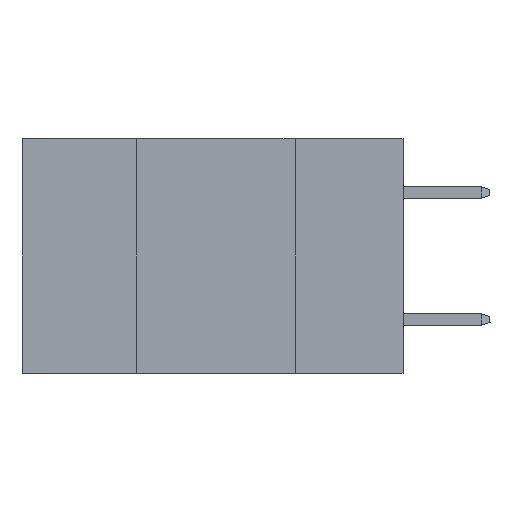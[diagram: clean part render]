
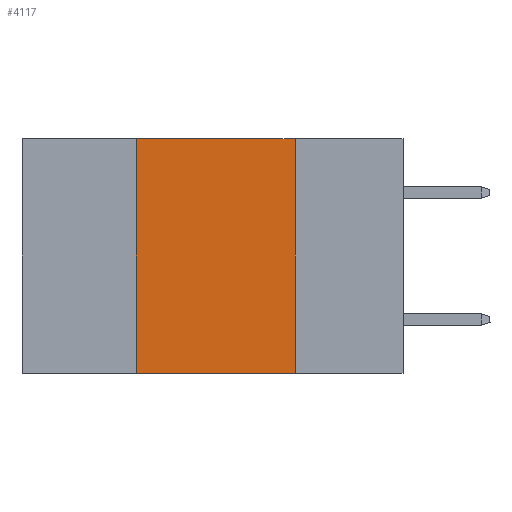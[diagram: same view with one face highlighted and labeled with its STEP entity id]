
A CAD part, left-side view. The second image highlights one B-rep face of the part: STEP entity #4117.
In plain terms, the highlighted planar face has unit normal (-1, 0, 0).
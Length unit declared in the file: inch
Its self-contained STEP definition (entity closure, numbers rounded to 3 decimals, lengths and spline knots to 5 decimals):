
#160 = FACE_OUTER_BOUND ( 'NONE', #6098, .T. ) ;
#969 = DIRECTION ( 'NONE',  ( 0., 0., -1. ) ) ;
#2615 = VERTEX_POINT ( 'NONE', #3359 ) ;
#2995 = LINE ( 'NONE', #11802, #12987 ) ;
#3111 = LINE ( 'NONE', #20006, #18843 ) ;
#3216 = PLANE ( 'NONE',  #6344 ) ;
#3313 = VERTEX_POINT ( 'NONE', #8486 ) ;
#3359 = CARTESIAN_POINT ( 'NONE',  ( 0., 0.42, 0. ) ) ;
#4117 = ADVANCED_FACE ( 'NONE', ( #160 ), #3216, .F. ) ;
#5046 = DIRECTION ( 'NONE',  ( 0., -1., 0. ) ) ;
#5376 = CARTESIAN_POINT ( 'NONE',  ( 0., 0.6, -0.37 ) ) ;
#5401 = CARTESIAN_POINT ( 'NONE',  ( 0., 0.42, -0.37 ) ) ;
#6098 = EDGE_LOOP ( 'NONE', ( #12849, #13222, #9980, #18121 ) ) ;
#6344 = AXIS2_PLACEMENT_3D ( 'NONE', #6979, #20107, #18427 ) ;
#6679 = VECTOR ( 'NONE', #969, 39.37008 ) ;
#6979 = CARTESIAN_POINT ( 'NONE',  ( 0., 0.6, 0. ) ) ;
#7390 = EDGE_CURVE ( 'NONE', #15322, #2615, #2995, .T. ) ;
#8486 = CARTESIAN_POINT ( 'NONE',  ( 0., 0.17, -0.37 ) ) ;
#9980 = ORIENTED_EDGE ( 'NONE', *, *, #7390, .F. ) ;
#11802 = CARTESIAN_POINT ( 'NONE',  ( 0., 0.42, 0. ) ) ;
#12151 = CARTESIAN_POINT ( 'NONE',  ( 0., 0.17, 0. ) ) ;
#12849 = ORIENTED_EDGE ( 'NONE', *, *, #13309, .F. ) ;
#12987 = VECTOR ( 'NONE', #19993, 39.37008 ) ;
#13222 = ORIENTED_EDGE ( 'NONE', *, *, #13305, .F. ) ;
#13290 = CARTESIAN_POINT ( 'NONE',  ( 0., 0.17, 0. ) ) ;
#13305 = EDGE_CURVE ( 'NONE', #2615, #20611, #3111, .T. ) ;
#13309 = EDGE_CURVE ( 'NONE', #20611, #3313, #21587, .T. ) ;
#14733 = DIRECTION ( 'NONE',  ( 0., -1., 0. ) ) ;
#15322 = VERTEX_POINT ( 'NONE', #5401 ) ;
#17035 = LINE ( 'NONE', #5376, #20017 ) ;
#18121 = ORIENTED_EDGE ( 'NONE', *, *, #18253, .T. ) ;
#18253 = EDGE_CURVE ( 'NONE', #15322, #3313, #17035, .T. ) ;
#18427 = DIRECTION ( 'NONE',  ( 0., 0., -1. ) ) ;
#18843 = VECTOR ( 'NONE', #14733, 39.37008 ) ;
#19993 = DIRECTION ( 'NONE',  ( 0., 0., 1. ) ) ;
#20006 = CARTESIAN_POINT ( 'NONE',  ( 0., 0.6, 0. ) ) ;
#20017 = VECTOR ( 'NONE', #5046, 39.37008 ) ;
#20107 = DIRECTION ( 'NONE',  ( 1., 0., 0. ) ) ;
#20611 = VERTEX_POINT ( 'NONE', #12151 ) ;
#21587 = LINE ( 'NONE', #13290, #6679 ) ;
